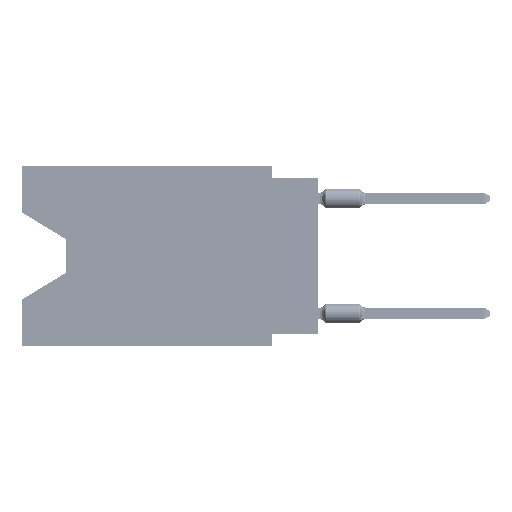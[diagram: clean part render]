
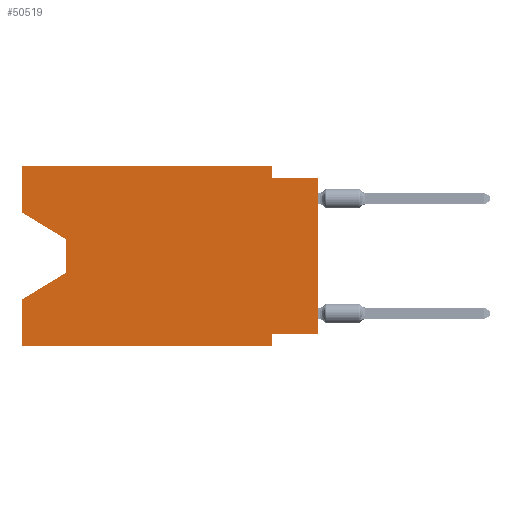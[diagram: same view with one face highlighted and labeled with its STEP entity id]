
A CAD part, left-side view. The second image highlights one B-rep face of the part: STEP entity #50519.
In plain terms, the highlighted planar face has unit normal (-1, 0, 0).
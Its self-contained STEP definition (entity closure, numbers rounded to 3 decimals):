
#1331 = DIRECTION ( 'NONE',  ( 0., 0.855, -0.519 ) ) ;
#2229 = PLANE ( 'NONE',  #9407 ) ;
#2571 = ORIENTED_EDGE ( 'NONE', *, *, #64121, .T. ) ;
#3817 = CARTESIAN_POINT ( 'NONE',  ( 0., 0., -9.271 ) ) ;
#5576 = LINE ( 'NONE', #52145, #6016 ) ;
#6016 = VECTOR ( 'NONE', #47136, 1000. ) ;
#6721 = CARTESIAN_POINT ( 'NONE',  ( 0., 13.97, -5.893 ) ) ;
#7432 = VECTOR ( 'NONE', #40148, 1000. ) ;
#7976 = LINE ( 'NONE', #12998, #25292 ) ;
#7991 = FACE_OUTER_BOUND ( 'NONE', #38945, .T. ) ;
#9407 = AXIS2_PLACEMENT_3D ( 'NONE', #49185, #72628, #68372 ) ;
#9756 = EDGE_CURVE ( 'NONE', #43332, #16981, #54362, .T. ) ;
#10574 = VECTOR ( 'NONE', #15393, 1000. ) ;
#10816 = ORIENTED_EDGE ( 'NONE', *, *, #25348, .T. ) ;
#11471 = VECTOR ( 'NONE', #1331, 1000. ) ;
#12615 = ORIENTED_EDGE ( 'NONE', *, *, #46486, .F. ) ;
#12998 = CARTESIAN_POINT ( 'NONE',  ( 0., 2.54, -9.906 ) ) ;
#13371 = CARTESIAN_POINT ( 'NONE',  ( 0., 16.383, 0. ) ) ;
#14546 = DIRECTION ( 'NONE',  ( 0., -1., 0. ) ) ;
#14860 = CARTESIAN_POINT ( 'NONE',  ( 0., 13.97, -4.013 ) ) ;
#15252 = VECTOR ( 'NONE', #31213, 1000. ) ;
#15393 = DIRECTION ( 'NONE',  ( 0., 0., 1. ) ) ;
#16981 = VERTEX_POINT ( 'NONE', #32636 ) ;
#17333 = CARTESIAN_POINT ( 'NONE',  ( 0., 16.383, -7.36 ) ) ;
#21081 = LINE ( 'NONE', #44174, #21956 ) ;
#21342 = EDGE_CURVE ( 'NONE', #34524, #39927, #56937, .T. ) ;
#21468 = EDGE_CURVE ( 'NONE', #57434, #43332, #59970, .T. ) ;
#21720 = VERTEX_POINT ( 'NONE', #27253 ) ;
#21956 = VECTOR ( 'NONE', #14546, 1000. ) ;
#22865 = CARTESIAN_POINT ( 'NONE',  ( 0., 13.97, -5.893 ) ) ;
#25292 = VECTOR ( 'NONE', #41890, 1000. ) ;
#25348 = EDGE_CURVE ( 'NONE', #49988, #39927, #42519, .T. ) ;
#26429 = ORIENTED_EDGE ( 'NONE', *, *, #49868, .T. ) ;
#27124 = LINE ( 'NONE', #50587, #67062 ) ;
#27253 = CARTESIAN_POINT ( 'NONE',  ( 0., 0., -0.635 ) ) ;
#28225 = CARTESIAN_POINT ( 'NONE',  ( 0., 16.383, 0. ) ) ;
#28453 = CARTESIAN_POINT ( 'NONE',  ( 0., 16.383, -2.546 ) ) ;
#28721 = VERTEX_POINT ( 'NONE', #28453 ) ;
#28760 = VERTEX_POINT ( 'NONE', #3817 ) ;
#29741 = CARTESIAN_POINT ( 'NONE',  ( 0., 0., 0. ) ) ;
#30068 = LINE ( 'NONE', #48134, #62972 ) ;
#30274 = VECTOR ( 'NONE', #30372, 1000. ) ;
#30299 = EDGE_CURVE ( 'NONE', #34524, #74794, #21081, .T. ) ;
#30372 = DIRECTION ( 'NONE',  ( 0., -1., 0. ) ) ;
#31213 = DIRECTION ( 'NONE',  ( 0., 0., -1. ) ) ;
#32636 = CARTESIAN_POINT ( 'NONE',  ( 0., 2.54, -0.635 ) ) ;
#34524 = VERTEX_POINT ( 'NONE', #70178 ) ;
#35471 = ORIENTED_EDGE ( 'NONE', *, *, #54515, .T. ) ;
#35473 = ORIENTED_EDGE ( 'NONE', *, *, #46446, .F. ) ;
#35491 = LINE ( 'NONE', #66197, #15252 ) ;
#37038 = VERTEX_POINT ( 'NONE', #58771 ) ;
#37227 = VERTEX_POINT ( 'NONE', #14860 ) ;
#37390 = EDGE_CURVE ( 'NONE', #16981, #21720, #5576, .T. ) ;
#37596 = VECTOR ( 'NONE', #59938, 1000. ) ;
#38945 = EDGE_LOOP ( 'NONE', ( #26429, #35471, #10816, #58178, #56853, #12615, #63030, #2571, #40381, #74235, #46913, #35473 ) ) ;
#39927 = VERTEX_POINT ( 'NONE', #17333 ) ;
#40148 = DIRECTION ( 'NONE',  ( 0., 0., 1. ) ) ;
#40381 = ORIENTED_EDGE ( 'NONE', *, *, #37390, .F. ) ;
#41286 = LINE ( 'NONE', #29741, #7432 ) ;
#41314 = DIRECTION ( 'NONE',  ( 0., 0., -1. ) ) ;
#41890 = DIRECTION ( 'NONE',  ( 0., 0., -1. ) ) ;
#42519 = LINE ( 'NONE', #6721, #11471 ) ;
#43332 = VERTEX_POINT ( 'NONE', #54560 ) ;
#44174 = CARTESIAN_POINT ( 'NONE',  ( 0., 16.383, -9.906 ) ) ;
#46446 = EDGE_CURVE ( 'NONE', #28721, #57434, #65319, .T. ) ;
#46486 = EDGE_CURVE ( 'NONE', #37038, #74794, #7976, .T. ) ;
#46913 = ORIENTED_EDGE ( 'NONE', *, *, #21468, .F. ) ;
#47136 = DIRECTION ( 'NONE',  ( 0., -1., 0. ) ) ;
#48134 = CARTESIAN_POINT ( 'NONE',  ( 0., 0., -9.271 ) ) ;
#49185 = CARTESIAN_POINT ( 'NONE',  ( 0., 16.383, 0. ) ) ;
#49868 = EDGE_CURVE ( 'NONE', #28721, #37227, #27124, .T. ) ;
#49988 = VERTEX_POINT ( 'NONE', #22865 ) ;
#50519 = ADVANCED_FACE ( 'NONE', ( #7991 ), #2229, .F. ) ;
#50587 = CARTESIAN_POINT ( 'NONE',  ( 0., 16.383, -2.546 ) ) ;
#52145 = CARTESIAN_POINT ( 'NONE',  ( 0., 0., -0.635 ) ) ;
#52311 = CARTESIAN_POINT ( 'NONE',  ( 0., 16.383, 0. ) ) ;
#54362 = LINE ( 'NONE', #64746, #65007 ) ;
#54515 = EDGE_CURVE ( 'NONE', #37227, #49988, #35491, .T. ) ;
#54560 = CARTESIAN_POINT ( 'NONE',  ( 0., 2.54, 0. ) ) ;
#56723 = DIRECTION ( 'NONE',  ( 0., -0.855, -0.519 ) ) ;
#56853 = ORIENTED_EDGE ( 'NONE', *, *, #30299, .T. ) ;
#56937 = LINE ( 'NONE', #68090, #10574 ) ;
#57434 = VERTEX_POINT ( 'NONE', #28225 ) ;
#58178 = ORIENTED_EDGE ( 'NONE', *, *, #21342, .F. ) ;
#58771 = CARTESIAN_POINT ( 'NONE',  ( 0., 2.54, -9.271 ) ) ;
#59938 = DIRECTION ( 'NONE',  ( 0., 0., 1. ) ) ;
#59970 = LINE ( 'NONE', #52311, #30274 ) ;
#62972 = VECTOR ( 'NONE', #70442, 1000. ) ;
#63030 = ORIENTED_EDGE ( 'NONE', *, *, #72899, .F. ) ;
#64121 = EDGE_CURVE ( 'NONE', #28760, #21720, #41286, .T. ) ;
#64746 = CARTESIAN_POINT ( 'NONE',  ( 0., 2.54, 0. ) ) ;
#65007 = VECTOR ( 'NONE', #41314, 1000. ) ;
#65319 = LINE ( 'NONE', #13371, #37596 ) ;
#66197 = CARTESIAN_POINT ( 'NONE',  ( 0., 13.97, -4.013 ) ) ;
#67062 = VECTOR ( 'NONE', #56723, 1000. ) ;
#68090 = CARTESIAN_POINT ( 'NONE',  ( 0., 16.383, 0. ) ) ;
#68372 = DIRECTION ( 'NONE',  ( 0., 0., -1. ) ) ;
#70178 = CARTESIAN_POINT ( 'NONE',  ( 0., 16.383, -9.906 ) ) ;
#70442 = DIRECTION ( 'NONE',  ( 0., 1., 0. ) ) ;
#70733 = CARTESIAN_POINT ( 'NONE',  ( 0., 2.54, -9.906 ) ) ;
#72628 = DIRECTION ( 'NONE',  ( 1., 0., 0. ) ) ;
#72899 = EDGE_CURVE ( 'NONE', #28760, #37038, #30068, .T. ) ;
#74235 = ORIENTED_EDGE ( 'NONE', *, *, #9756, .F. ) ;
#74794 = VERTEX_POINT ( 'NONE', #70733 ) ;
